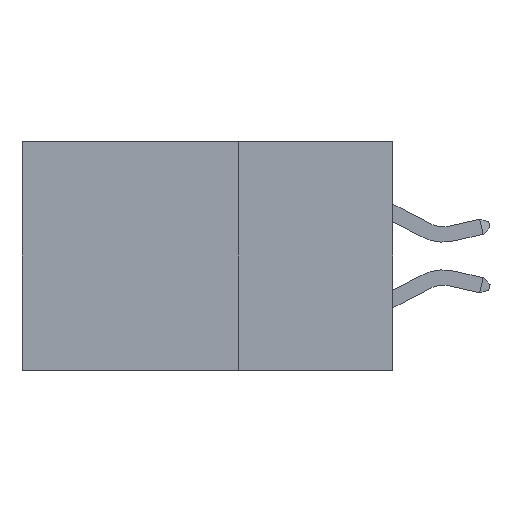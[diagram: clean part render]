
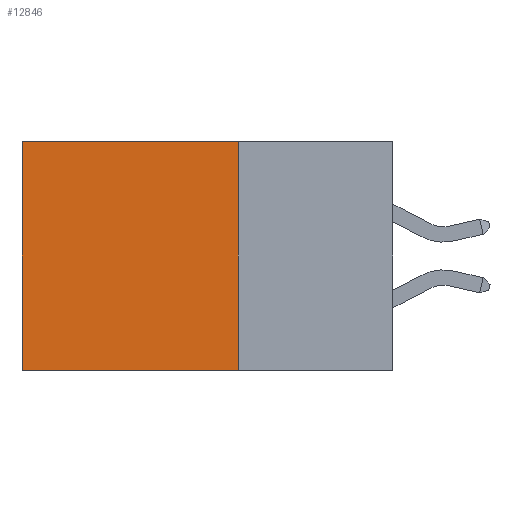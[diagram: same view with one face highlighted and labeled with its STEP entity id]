
A CAD part, left-side view. The second image highlights one B-rep face of the part: STEP entity #12846.
In plain terms, the highlighted planar face has unit normal (-1, 0, 0).
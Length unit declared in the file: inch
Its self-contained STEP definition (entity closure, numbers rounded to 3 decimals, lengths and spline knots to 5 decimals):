
#794 = VERTEX_POINT ( 'NONE', #18064 ) ;
#1187 = FACE_OUTER_BOUND ( 'NONE', #16623, .T. ) ;
#1737 = LINE ( 'NONE', #18688, #9177 ) ;
#2108 = ORIENTED_EDGE ( 'NONE', *, *, #14756, .F. ) ;
#2412 = AXIS2_PLACEMENT_3D ( 'NONE', #8842, #18874, #10330 ) ;
#2852 = DIRECTION ( 'NONE',  ( 0., 0., -1. ) ) ;
#3153 = CARTESIAN_POINT ( 'NONE',  ( 0.2875, 0.25, -0.37 ) ) ;
#3562 = VECTOR ( 'NONE', #10900, 39.37008 ) ;
#4814 = VECTOR ( 'NONE', #10565, 39.37008 ) ;
#5394 = EDGE_CURVE ( 'NONE', #794, #17346, #1737, .T. ) ;
#6190 = VERTEX_POINT ( 'NONE', #3153 ) ;
#6505 = ORIENTED_EDGE ( 'NONE', *, *, #11295, .T. ) ;
#6726 = VECTOR ( 'NONE', #17861, 39.37008 ) ;
#7217 = LINE ( 'NONE', #9243, #6726 ) ;
#8316 = LINE ( 'NONE', #17706, #4814 ) ;
#8842 = CARTESIAN_POINT ( 'NONE',  ( 0.2875, 0.25, 0. ) ) ;
#9177 = VECTOR ( 'NONE', #2852, 39.37008 ) ;
#9243 = CARTESIAN_POINT ( 'NONE',  ( 0.2875, 0.25, 0. ) ) ;
#10330 = DIRECTION ( 'NONE',  ( 0., 0., -1. ) ) ;
#10565 = DIRECTION ( 'NONE',  ( 0., 1., 0. ) ) ;
#10784 = VERTEX_POINT ( 'NONE', #11301 ) ;
#10836 = CARTESIAN_POINT ( 'NONE',  ( 0.2875, 0.25, 0. ) ) ;
#10900 = DIRECTION ( 'NONE',  ( 0., 1., 0. ) ) ;
#11295 = EDGE_CURVE ( 'NONE', #10784, #794, #15707, .T. ) ;
#11301 = CARTESIAN_POINT ( 'NONE',  ( 0.2875, 0.25, 0. ) ) ;
#12846 = ADVANCED_FACE ( 'NONE', ( #1187 ), #17481, .F. ) ;
#13605 = EDGE_CURVE ( 'NONE', #10784, #6190, #7217, .T. ) ;
#14411 = CARTESIAN_POINT ( 'NONE',  ( 0.2875, 0.6, -0.37 ) ) ;
#14756 = EDGE_CURVE ( 'NONE', #6190, #17346, #8316, .T. ) ;
#15554 = ORIENTED_EDGE ( 'NONE', *, *, #13605, .F. ) ;
#15707 = LINE ( 'NONE', #10836, #3562 ) ;
#16623 = EDGE_LOOP ( 'NONE', ( #16963, #2108, #15554, #6505 ) ) ;
#16963 = ORIENTED_EDGE ( 'NONE', *, *, #5394, .T. ) ;
#17346 = VERTEX_POINT ( 'NONE', #14411 ) ;
#17481 = PLANE ( 'NONE',  #2412 ) ;
#17706 = CARTESIAN_POINT ( 'NONE',  ( 0.2875, 0.25, -0.37 ) ) ;
#17861 = DIRECTION ( 'NONE',  ( 0., 0., -1. ) ) ;
#18064 = CARTESIAN_POINT ( 'NONE',  ( 0.2875, 0.6, 0. ) ) ;
#18688 = CARTESIAN_POINT ( 'NONE',  ( 0.2875, 0.6, 0. ) ) ;
#18874 = DIRECTION ( 'NONE',  ( 1., 0., 0. ) ) ;
